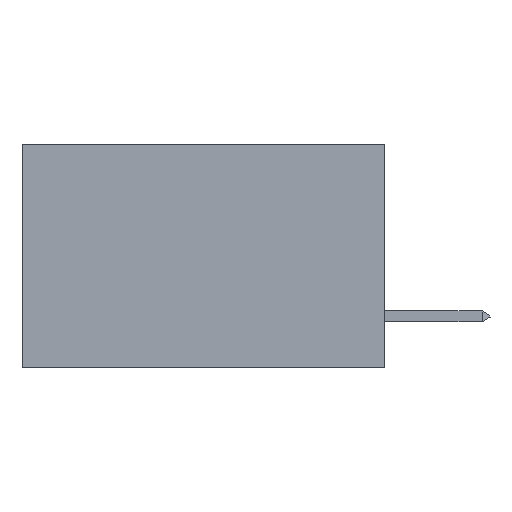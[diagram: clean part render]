
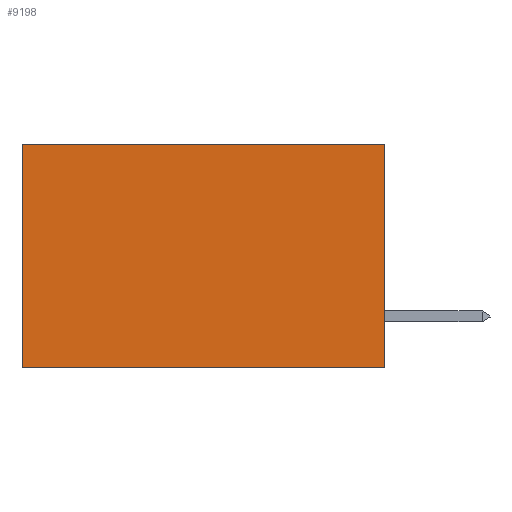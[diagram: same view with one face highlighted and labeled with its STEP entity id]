
A CAD part, left-side view. The second image highlights one B-rep face of the part: STEP entity #9198.
In plain terms, the highlighted planar face has unit normal (-1, 0, 0).
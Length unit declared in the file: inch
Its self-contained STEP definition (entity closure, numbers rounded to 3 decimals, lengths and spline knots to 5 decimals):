
#82 = CARTESIAN_POINT ( 'NONE',  ( 0.2875, 0., -0.37 ) ) ;
#178 = EDGE_CURVE ( 'NONE', #1121, #879, #3080, .T. ) ;
#879 = VERTEX_POINT ( 'NONE', #9213 ) ;
#1121 = VERTEX_POINT ( 'NONE', #7011 ) ;
#1490 = EDGE_CURVE ( 'NONE', #2738, #1121, #1670, .T. ) ;
#1670 = LINE ( 'NONE', #11783, #11446 ) ;
#2138 = FACE_OUTER_BOUND ( 'NONE', #9304, .T. ) ;
#2289 = PLANE ( 'NONE',  #16611 ) ;
#2405 = DIRECTION ( 'NONE',  ( 1., 0., 0. ) ) ;
#2443 = LINE ( 'NONE', #5912, #4589 ) ;
#2738 = VERTEX_POINT ( 'NONE', #7779 ) ;
#3080 = LINE ( 'NONE', #82, #10080 ) ;
#3378 = EDGE_CURVE ( 'NONE', #2738, #6949, #14014, .T. ) ;
#4018 = DIRECTION ( 'NONE',  ( 0., 1., 0. ) ) ;
#4095 = DIRECTION ( 'NONE',  ( 0., 0., -1. ) ) ;
#4589 = VECTOR ( 'NONE', #8579, 39.37008 ) ;
#5043 = CARTESIAN_POINT ( 'NONE',  ( 0.2875, 0.6, 0. ) ) ;
#5231 = ORIENTED_EDGE ( 'NONE', *, *, #1490, .F. ) ;
#5912 = CARTESIAN_POINT ( 'NONE',  ( 0.2875, 0.6, 0. ) ) ;
#6594 = DIRECTION ( 'NONE',  ( 0., 0., -1. ) ) ;
#6632 = EDGE_CURVE ( 'NONE', #6949, #879, #2443, .T. ) ;
#6949 = VERTEX_POINT ( 'NONE', #5043 ) ;
#7011 = CARTESIAN_POINT ( 'NONE',  ( 0.2875, 0., -0.37 ) ) ;
#7779 = CARTESIAN_POINT ( 'NONE',  ( 0.2875, 0., 0. ) ) ;
#8579 = DIRECTION ( 'NONE',  ( 0., 0., -1. ) ) ;
#9198 = ADVANCED_FACE ( 'NONE', ( #2138 ), #2289, .F. ) ;
#9213 = CARTESIAN_POINT ( 'NONE',  ( 0.2875, 0.6, -0.37 ) ) ;
#9304 = EDGE_LOOP ( 'NONE', ( #11347, #14303, #5231, #10424 ) ) ;
#10080 = VECTOR ( 'NONE', #4018, 39.37008 ) ;
#10424 = ORIENTED_EDGE ( 'NONE', *, *, #3378, .T. ) ;
#11347 = ORIENTED_EDGE ( 'NONE', *, *, #6632, .T. ) ;
#11446 = VECTOR ( 'NONE', #4095, 39.37008 ) ;
#11561 = CARTESIAN_POINT ( 'NONE',  ( 0.2875, 0., 0. ) ) ;
#11783 = CARTESIAN_POINT ( 'NONE',  ( 0.2875, 0., 0. ) ) ;
#12994 = VECTOR ( 'NONE', #14278, 39.37008 ) ;
#14014 = LINE ( 'NONE', #11561, #12994 ) ;
#14278 = DIRECTION ( 'NONE',  ( 0., 1., 0. ) ) ;
#14303 = ORIENTED_EDGE ( 'NONE', *, *, #178, .F. ) ;
#16611 = AXIS2_PLACEMENT_3D ( 'NONE', #16637, #2405, #6594 ) ;
#16637 = CARTESIAN_POINT ( 'NONE',  ( 0.2875, 0., 0. ) ) ;
